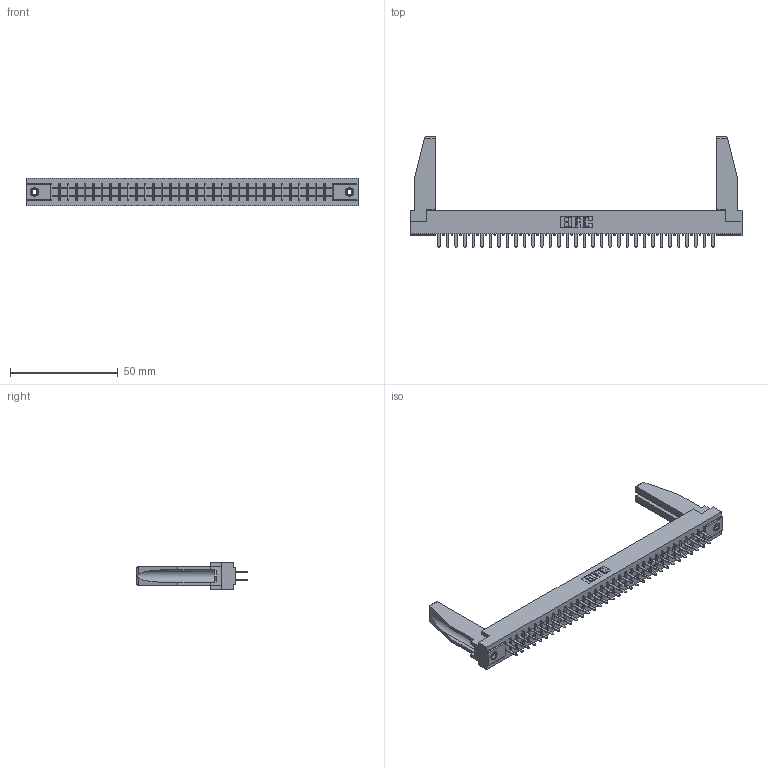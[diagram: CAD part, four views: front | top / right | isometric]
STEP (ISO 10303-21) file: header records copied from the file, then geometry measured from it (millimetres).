
FILE_DESCRIPTION (( 'STEP AP203' ), '1' );
FILE_NAME ('355-066-520-278.STEP', '2019-09-12T15:32:28', ( '' ), ( '' ), 'SwSTEP 2.0', 'SolidWorks 2016', '' );
FILE_SCHEMA (( 'CONFIG_CONTROL_DESIGN' ));
Length unit declared in the file: inch
Products named in the file (5): 355-066-520-278; 345-250-001_345-250-001-102; 305-290-001_520; 307-220-078; 305 Part_.156 Dia
Assembly tree (71 placements, depth 2):
  355-066-520-278
    305 Part_.156 Dia
    305-290-001_520  x66
    345-250-001_345-250-001-102  x2
    307-220-078  x2
Bounding box: 153.77 x 51.13 x 12.7 mm (x, y, z)
Volume: 19971 mm3; surface area: 24007.6 mm2
Topology: 71 solids, 71 shells, 3282 faces, 9325 edges, 6030 vertices
Faces by surface type: plane 1934, cylinder 1200, sphere 132, cone 12, torus 4
Entity records: 39145 total; most frequent: CARTESIAN_POINT 6483, ORIENTED_EDGE 6392, DIRECTION 6236, EDGE_CURVE 3196, LINE 2574, VECTOR 2574, VERTEX_POINT 2036, AXIS2_PLACEMENT_3D 1831
